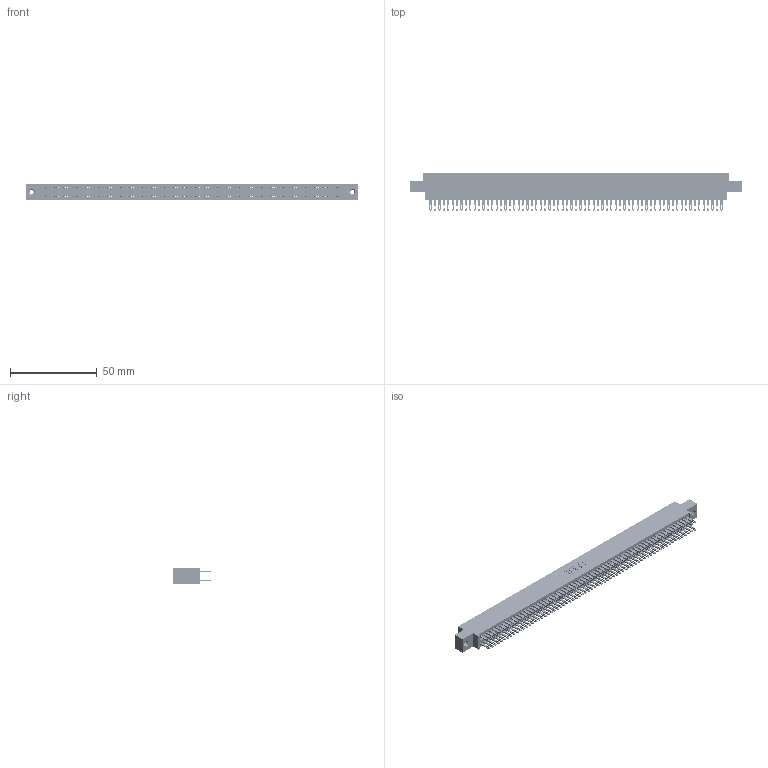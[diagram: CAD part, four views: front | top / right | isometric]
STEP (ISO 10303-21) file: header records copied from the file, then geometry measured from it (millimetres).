
FILE_DESCRIPTION (( 'STEP AP203' ), '1' );
FILE_NAME ('345-134-500-807.STEP', '2019-11-08T00:09:39', ( '' ), ( '' ), 'SwSTEP 2.0', 'SolidWorks 2016', '' );
FILE_SCHEMA (( 'CONFIG_CONTROL_DESIGN' ));
Length unit declared in the file: inch
Products named in the file (4): 345-134-500-807; 345 Part_0.170 Offset - 0.156 Dia-TI; 345-250-001_345-250-005-103; 345-292-001_345-293-100
Assembly tree (137 placements, depth 2):
  345-134-500-807
    345 Part_0.170 Offset - 0.156 Dia-TI
    345-292-001_345-293-100  x134
    345-250-001_345-250-005-103  x2
Bounding box: 191.39 x 21.51 x 9.4 mm (x, y, z)
Volume: 19106.4 mm3; surface area: 30264.7 mm2
Topology: 137 solids, 137 shells, 6354 faces, 19383 edges, 12914 vertices
Faces by surface type: plane 3734, cylinder 2604, cone 12, torus 4
Entity records: 50452 total; most frequent: CARTESIAN_POINT 8415, ORIENTED_EDGE 8342, DIRECTION 7417, EDGE_CURVE 4171, LINE 3747, VECTOR 3747, VERTEX_POINT 2776, AXIS2_PLACEMENT_3D 1835
